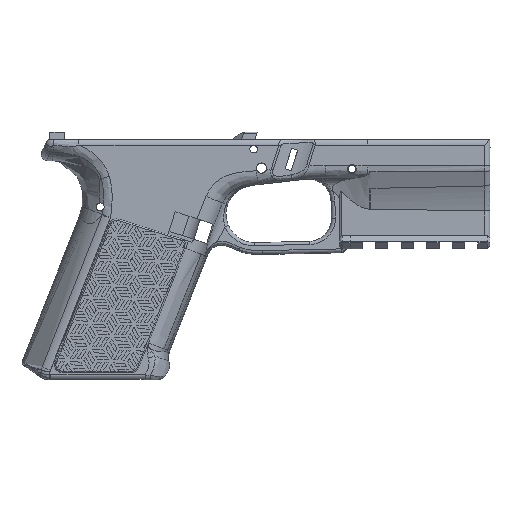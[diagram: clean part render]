
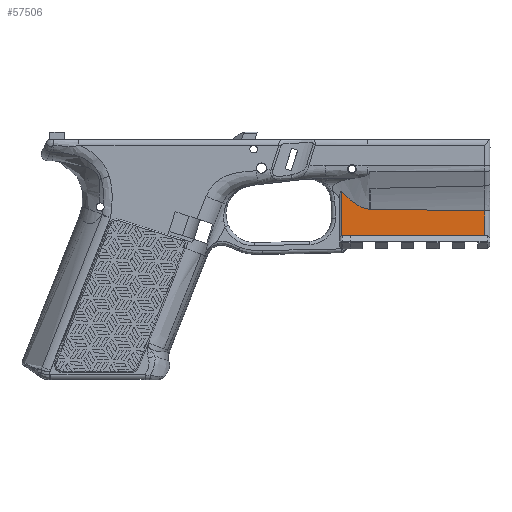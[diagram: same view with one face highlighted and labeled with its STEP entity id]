
A CAD part, top view. The second image highlights one B-rep face of the part: STEP entity #57506.
In plain terms, the highlighted planar face has unit normal (0, 0, 1).
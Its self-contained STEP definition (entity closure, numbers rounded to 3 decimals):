
#2386=(
BOUNDED_CURVE()
B_SPLINE_CURVE(2,(#126953,#126954,#126955),.UNSPECIFIED.,.F.,.F.)
B_SPLINE_CURVE_WITH_KNOTS((3,3),(0.033,4.501),
 .UNSPECIFIED.)
CURVE()
GEOMETRIC_REPRESENTATION_ITEM()
RATIONAL_B_SPLINE_CURVE((1.,1.,1.))
REPRESENTATION_ITEM('')
);
#8819=LINE('',#126619,#14013);
#8836=LINE('',#126959,#14030);
#8837=LINE('',#126966,#14031);
#14013=VECTOR('',#69991,10.);
#14030=VECTOR('',#70040,10.);
#14031=VECTOR('',#70043,10.);
#15662=PLANE('',#60003);
#15865=B_SPLINE_CURVE_WITH_KNOTS('',3,(#105134,#105135,#105136,#105137,
#105138,#105139),.UNSPECIFIED.,.F.,.F.,(4,2,4),(-0.021,-0.011,
0.),.UNSPECIFIED.);
#15867=B_SPLINE_CURVE_WITH_KNOTS('',3,(#105192,#105193,#105194,#105195,
#105196,#105197,#105198,#105199),.UNSPECIFIED.,.F.,.F.,(4,2,2,4),(-0.895,
-0.59,-0.274,0.),.UNSPECIFIED.);
#16207=B_SPLINE_CURVE_WITH_KNOTS('',3,(#126960,#126961,#126962,#126963),
 .UNSPECIFIED.,.F.,.F.,(4,4),(-0.905,-0.904),
 .UNSPECIFIED.);
#19300=FACE_OUTER_BOUND('',#22656,.T.);
#22656=EDGE_LOOP('',(#53931,#53932,#53933,#53934,#53935,#53936,#53937,#53938));
#23359=CIRCLE('',#60004,1.);
#27952=VERTEX_POINT('',#105132);
#27953=VERTEX_POINT('',#105133);
#27956=VERTEX_POINT('',#105173);
#28816=VERTEX_POINT('',#126618);
#28834=VERTEX_POINT('',#126951);
#28835=VERTEX_POINT('',#126957);
#28836=VERTEX_POINT('',#126958);
#28837=VERTEX_POINT('',#126964);
#35788=EDGE_CURVE('',#27952,#27953,#15865,.T.);
#35793=EDGE_CURVE('',#27956,#27952,#15867,.T.);
#37208=EDGE_CURVE('',#28816,#27956,#8819,.T.);
#37241=EDGE_CURVE('',#27953,#28834,#2386,.T.);
#37242=EDGE_CURVE('',#28835,#28836,#8836,.T.);
#37243=EDGE_CURVE('',#28834,#28835,#16207,.T.);
#37244=EDGE_CURVE('',#28816,#28837,#23359,.T.);
#37245=EDGE_CURVE('',#28836,#28837,#8837,.T.);
#53931=ORIENTED_EDGE('',*,*,#37242,.F.);
#53932=ORIENTED_EDGE('',*,*,#37243,.F.);
#53933=ORIENTED_EDGE('',*,*,#37241,.F.);
#53934=ORIENTED_EDGE('',*,*,#35788,.F.);
#53935=ORIENTED_EDGE('',*,*,#35793,.F.);
#53936=ORIENTED_EDGE('',*,*,#37208,.F.);
#53937=ORIENTED_EDGE('',*,*,#37244,.T.);
#53938=ORIENTED_EDGE('',*,*,#37245,.F.);
#57506=ADVANCED_FACE('',(#19300),#15662,.T.);
#60003=AXIS2_PLACEMENT_3D('',#126956,#70038,#70039);
#60004=AXIS2_PLACEMENT_3D('',#126965,#70041,#70042);
#69991=DIRECTION('',(0.,1.,0.));
#70038=DIRECTION('center_axis',(0.,0.,
1.));
#70039=DIRECTION('ref_axis',(1.,0.,0.));
#70040=DIRECTION('',(0.,-1.,0.));
#70041=DIRECTION('center_axis',(0.,0.,
-1.));
#70042=DIRECTION('ref_axis',(-0.707,0.707,0.));
#70043=DIRECTION('',(-1.,0.,0.));
#105132=CARTESIAN_POINT('',(125.329,-28.666,8.018));
#105133=CARTESIAN_POINT('',(125.539,-28.671,8.018));
#105134=CARTESIAN_POINT('Ctrl Pts',(125.329,-28.666,
8.018));
#105135=CARTESIAN_POINT('Ctrl Pts',(125.364,-28.667,
8.018));
#105136=CARTESIAN_POINT('Ctrl Pts',(125.399,-28.668,8.018));
#105137=CARTESIAN_POINT('Ctrl Pts',(125.469,-28.67,
8.018));
#105138=CARTESIAN_POINT('Ctrl Pts',(125.504,-28.671,
8.018));
#105139=CARTESIAN_POINT('Ctrl Pts',(125.539,-28.671,
8.018));
#105173=CARTESIAN_POINT('',(114.151,-21.776,8.018));
#105192=CARTESIAN_POINT('Ctrl Pts',(114.151,-21.776,
8.018));
#105193=CARTESIAN_POINT('Ctrl Pts',(115.249,-22.99,
8.018));
#105194=CARTESIAN_POINT('Ctrl Pts',(116.433,-24.15,
8.018));
#105195=CARTESIAN_POINT('Ctrl Pts',(118.978,-26.227,
8.018));
#105196=CARTESIAN_POINT('Ctrl Pts',(120.444,-27.212,
8.018));
#105197=CARTESIAN_POINT('Ctrl Pts',(123.311,-28.433,
8.018));
#105198=CARTESIAN_POINT('Ctrl Pts',(124.415,-28.63,8.018));
#105199=CARTESIAN_POINT('Ctrl Pts',(125.329,-28.666,
8.018));
#126618=CARTESIAN_POINT('',(114.151,-39.144,8.018));
#126619=CARTESIAN_POINT('',(114.151,-39.479,8.018));
#126951=CARTESIAN_POINT('',(170.327,-29.345,8.018));
#126953=CARTESIAN_POINT('Ctrl Pts',(125.539,-28.671,
8.018));
#126954=CARTESIAN_POINT('Ctrl Pts',(149.167,-28.978,
8.018));
#126955=CARTESIAN_POINT('Ctrl Pts',(170.327,-29.345,
8.018));
#126956=CARTESIAN_POINT('Origin',(134.968,-34.819,8.018));
#126957=CARTESIAN_POINT('',(170.336,-29.345,8.018));
#126958=CARTESIAN_POINT('',(170.336,-39.06,8.018));
#126959=CARTESIAN_POINT('',(170.336,-39.479,8.018));
#126960=CARTESIAN_POINT('Ctrl Pts',(170.327,-29.345,
8.018));
#126961=CARTESIAN_POINT('Ctrl Pts',(170.33,-29.345,
8.018));
#126962=CARTESIAN_POINT('Ctrl Pts',(170.333,-29.345,
8.018));
#126963=CARTESIAN_POINT('Ctrl Pts',(170.336,-29.345,8.018));
#126964=CARTESIAN_POINT('',(114.551,-39.06,8.018));
#126965=CARTESIAN_POINT('Origin',(114.551,-40.06,8.018));
#126966=CARTESIAN_POINT('',(117.551,-39.06,8.018));
